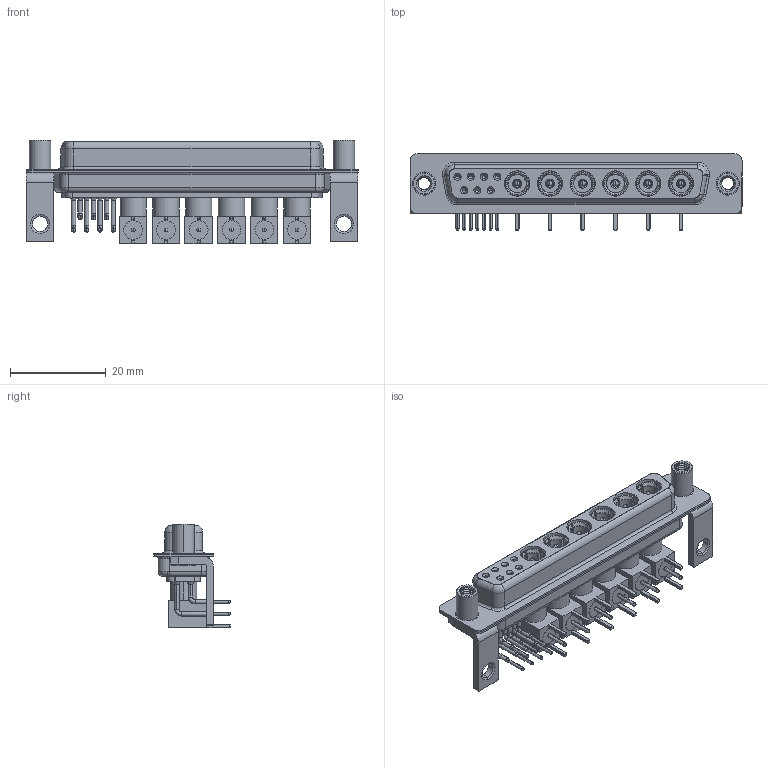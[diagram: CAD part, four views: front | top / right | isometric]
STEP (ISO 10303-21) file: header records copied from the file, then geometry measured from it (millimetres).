
FILE_DESCRIPTION (( 'STEP AP203' ), '1' );
FILE_NAME ('630-13W6640-5N6.STEP', '2022-06-06T15:15:36', ( '' ), ( '' ), 'SwSTEP 2.0', 'SolidWorks 2020', '' );
FILE_SCHEMA (( 'CONFIG_CONTROL_DESIGN' ));
Length unit declared in the file: millimetre
Products named in the file (20): Co-Ax Plug Assy_RA; 630Combo Stabilizer Bracket; 630Combo Threaded Standoff_D; Insulator Pin_Straight PC Tail; 630Combo Contact Row 1; Locking Collar; RA Back Shell; 630Combo Housing_13W6; Insulator RA Pin; 630-13W6640-5N6; 630Combo Contact Row 2; Pin_RA; 630Combo Shell Front_37 Contacts; Co-Ax Plug_RA PC Tail; 630Combo Shell Rear_37 Contacts
Assembly tree (56 placements, depth 3):
  630-13W6640-5N6
    630Combo Housing_13W6
    630Combo Shell Front_37 Contacts
    630Combo Shell Rear_37 Contacts
    630Combo Stabilizer Bracket  x2
    630Combo Threaded Standoff_D  x2
    Co-Ax Plug Assy_RA
      Co-Ax Plug_RA PC Tail
      Insulator Pin_Straight PC Tail
      Pin_RA
      Locking Collar
      RA Back Shell
      Insulator RA Pin
    Co-Ax Plug Assy_RA
      Co-Ax Plug_RA PC Tail
      Insulator Pin_Straight PC Tail
      Pin_RA
      Locking Collar
      RA Back Shell
      Insulator RA Pin
    Co-Ax Plug Assy_RA
      Co-Ax Plug_RA PC Tail
      Insulator Pin_Straight PC Tail
      Pin_RA
      Locking Collar
      RA Back Shell
      Insulator RA Pin
    Co-Ax Plug Assy_RA
      Co-Ax Plug_RA PC Tail
      Insulator Pin_Straight PC Tail
      Pin_RA
      Locking Collar
      RA Back Shell
      Insulator RA Pin
    Co-Ax Plug Assy_RA
      Co-Ax Plug_RA PC Tail
      Insulator Pin_Straight PC Tail
      Pin_RA
      Locking Collar
      RA Back Shell
      Insulator RA Pin
    Co-Ax Plug Assy_RA
      Co-Ax Plug_RA PC Tail
      Insulator Pin_Straight PC Tail
      Pin_RA
      Locking Collar
      RA Back Shell
      Insulator RA Pin
    630Combo Contact Row 1  x4
    630Combo Contact Row 2  x3
Bounding box: 69.4 x 16 x 21.61 mm (x, y, z)
Volume: 7053.5 mm3; surface area: 16879.8 mm2
Topology: 50 solids, 50 shells, 1756 faces, 4306 edges, 2706 vertices
Faces by surface type: cylinder 760, plane 596, cone 243, torus 93, bspline 40, sphere 24
Entity records: 25311 total; most frequent: CARTESIAN_POINT 6252, DIRECTION 3610, ORIENTED_EDGE 3180, EDGE_CURVE 1590, AXIS2_PLACEMENT_3D 1470, VERTEX_POINT 1013, EDGE_LOOP 767, CIRCLE 758
